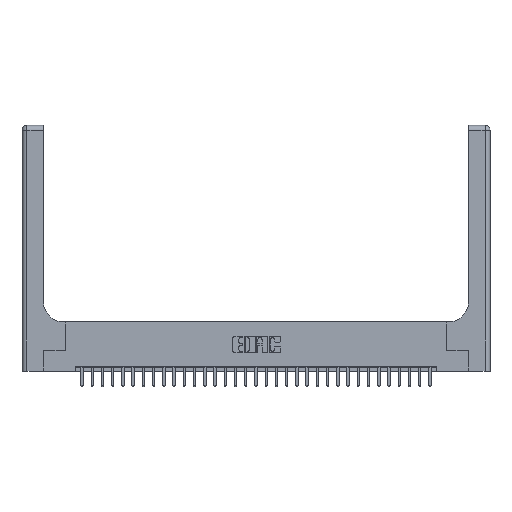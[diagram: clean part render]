
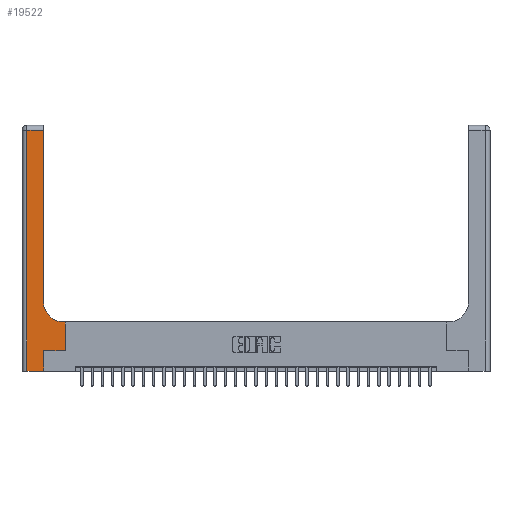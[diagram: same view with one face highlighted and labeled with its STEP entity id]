
A CAD part, top view. The second image highlights one B-rep face of the part: STEP entity #19522.
In plain terms, the highlighted planar face has unit normal (0, 0, 1).
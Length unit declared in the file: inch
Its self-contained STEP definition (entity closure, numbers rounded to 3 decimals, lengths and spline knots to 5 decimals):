
#517 = CARTESIAN_POINT ( 'NONE',  ( 0.265, 0., 0.37 ) ) ;
#1411 = CARTESIAN_POINT ( 'NONE',  ( 0.51, 0.6, 0.37 ) ) ;
#1595 = CARTESIAN_POINT ( 'NONE',  ( 0.06, 0., 0.37 ) ) ;
#1991 = VERTEX_POINT ( 'NONE', #1411 ) ;
#2302 = CARTESIAN_POINT ( 'NONE',  ( 0.528, 0.6, 0.37 ) ) ;
#2809 = CARTESIAN_POINT ( 'NONE',  ( 0., 2.94, 0.37 ) ) ;
#3441 = EDGE_LOOP ( 'NONE', ( #17980, #3738, #21100, #5610, #10237, #23819, #13665, #9428, #19962 ) ) ;
#3738 = ORIENTED_EDGE ( 'NONE', *, *, #18465, .T. ) ;
#3792 = EDGE_CURVE ( 'NONE', #15348, #22549, #23610, .T. ) ;
#4317 = DIRECTION ( 'NONE',  ( 0., 0., -1. ) ) ;
#4508 = DIRECTION ( 'NONE',  ( 0., 1., 0. ) ) ;
#5221 = EDGE_CURVE ( 'NONE', #27027, #10952, #20369, .T. ) ;
#5231 = DIRECTION ( 'NONE',  ( 1., 0., 0. ) ) ;
#5459 = CARTESIAN_POINT ( 'NONE',  ( 0.26, 0.85, 0.37 ) ) ;
#5610 = ORIENTED_EDGE ( 'NONE', *, *, #14222, .T. ) ;
#5787 = CARTESIAN_POINT ( 'NONE',  ( 0.265, 0., 0.37 ) ) ;
#6041 = VERTEX_POINT ( 'NONE', #15601 ) ;
#6692 = VECTOR ( 'NONE', #4508, 39.37008 ) ;
#7162 = LINE ( 'NONE', #14591, #27572 ) ;
#7606 = CARTESIAN_POINT ( 'NONE',  ( 0.26, 0.6, 0.37 ) ) ;
#8074 = VECTOR ( 'NONE', #21569, 39.37008 ) ;
#8231 = DIRECTION ( 'NONE',  ( -1., 0., 0. ) ) ;
#8663 = DIRECTION ( 'NONE',  ( 0., 1., 0. ) ) ;
#8794 = CARTESIAN_POINT ( 'NONE',  ( 0.528, 0.25, 0.37 ) ) ;
#9054 = CARTESIAN_POINT ( 'NONE',  ( 0.528, 0.25, 0.37 ) ) ;
#9428 = ORIENTED_EDGE ( 'NONE', *, *, #15849, .T. ) ;
#9912 = LINE ( 'NONE', #7606, #10601 ) ;
#10237 = ORIENTED_EDGE ( 'NONE', *, *, #17743, .T. ) ;
#10290 = DIRECTION ( 'NONE',  ( 1., 0., 0. ) ) ;
#10337 = VERTEX_POINT ( 'NONE', #5459 ) ;
#10601 = VECTOR ( 'NONE', #18874, 39.37008 ) ;
#10797 = CARTESIAN_POINT ( 'NONE',  ( 0.06, 3., 0.37 ) ) ;
#10952 = VERTEX_POINT ( 'NONE', #2302 ) ;
#11140 = EDGE_CURVE ( 'NONE', #1991, #10337, #25987, .T. ) ;
#11217 = PLANE ( 'NONE',  #22877 ) ;
#11635 = VECTOR ( 'NONE', #15423, 39.37008 ) ;
#11756 = DIRECTION ( 'NONE',  ( 1., 0., 0. ) ) ;
#12566 = CARTESIAN_POINT ( 'NONE',  ( 0.265, 0.25, 0.37 ) ) ;
#13026 = LINE ( 'NONE', #28829, #24299 ) ;
#13665 = ORIENTED_EDGE ( 'NONE', *, *, #5221, .T. ) ;
#14222 = EDGE_CURVE ( 'NONE', #22549, #14985, #7162, .T. ) ;
#14378 = VECTOR ( 'NONE', #8231, 39.37008 ) ;
#14591 = CARTESIAN_POINT ( 'NONE',  ( 0., 0., 0.37 ) ) ;
#14985 = VERTEX_POINT ( 'NONE', #517 ) ;
#15054 = LINE ( 'NONE', #2809, #14378 ) ;
#15348 = VERTEX_POINT ( 'NONE', #19340 ) ;
#15423 = DIRECTION ( 'NONE',  ( 0., -1., 0. ) ) ;
#15440 = LINE ( 'NONE', #5787, #8074 ) ;
#15601 = CARTESIAN_POINT ( 'NONE',  ( 0.26, 2.94, 0.37 ) ) ;
#15849 = EDGE_CURVE ( 'NONE', #10952, #1991, #9912, .T. ) ;
#17743 = EDGE_CURVE ( 'NONE', #14985, #22910, #15440, .T. ) ;
#17980 = ORIENTED_EDGE ( 'NONE', *, *, #26905, .T. ) ;
#18465 = EDGE_CURVE ( 'NONE', #6041, #15348, #15054, .T. ) ;
#18529 = CARTESIAN_POINT ( 'NONE',  ( 0.51, 0.85, 0.37 ) ) ;
#18874 = DIRECTION ( 'NONE',  ( -1., 0., 0. ) ) ;
#19340 = CARTESIAN_POINT ( 'NONE',  ( 0.06, 2.94, 0.37 ) ) ;
#19522 = ADVANCED_FACE ( 'NONE', ( #25866 ), #11217, .F. ) ;
#19962 = ORIENTED_EDGE ( 'NONE', *, *, #11140, .T. ) ;
#20341 = EDGE_CURVE ( 'NONE', #22910, #27027, #23754, .T. ) ;
#20369 = LINE ( 'NONE', #8794, #6692 ) ;
#20471 = AXIS2_PLACEMENT_3D ( 'NONE', #18529, #21107, #11756 ) ;
#21100 = ORIENTED_EDGE ( 'NONE', *, *, #3792, .T. ) ;
#21107 = DIRECTION ( 'NONE',  ( 0., 0., -1. ) ) ;
#21569 = DIRECTION ( 'NONE',  ( 0., 1., 0. ) ) ;
#22260 = DIRECTION ( 'NONE',  ( -1., 0., 0. ) ) ;
#22549 = VERTEX_POINT ( 'NONE', #1595 ) ;
#22877 = AXIS2_PLACEMENT_3D ( 'NONE', #27101, #4317, #22260 ) ;
#22910 = VERTEX_POINT ( 'NONE', #24541 ) ;
#23610 = LINE ( 'NONE', #10797, #11635 ) ;
#23754 = LINE ( 'NONE', #12566, #28341 ) ;
#23819 = ORIENTED_EDGE ( 'NONE', *, *, #20341, .T. ) ;
#24299 = VECTOR ( 'NONE', #8663, 39.37008 ) ;
#24541 = CARTESIAN_POINT ( 'NONE',  ( 0.265, 0.25, 0.37 ) ) ;
#25866 = FACE_OUTER_BOUND ( 'NONE', #3441, .T. ) ;
#25987 = CIRCLE ( 'NONE', #20471, 0.25 ) ;
#26905 = EDGE_CURVE ( 'NONE', #10337, #6041, #13026, .T. ) ;
#27027 = VERTEX_POINT ( 'NONE', #9054 ) ;
#27101 = CARTESIAN_POINT ( 'NONE',  ( 0., 3., 0.37 ) ) ;
#27572 = VECTOR ( 'NONE', #5231, 39.37008 ) ;
#28341 = VECTOR ( 'NONE', #10290, 39.37008 ) ;
#28829 = CARTESIAN_POINT ( 'NONE',  ( 0.26, 3., 0.37 ) ) ;
